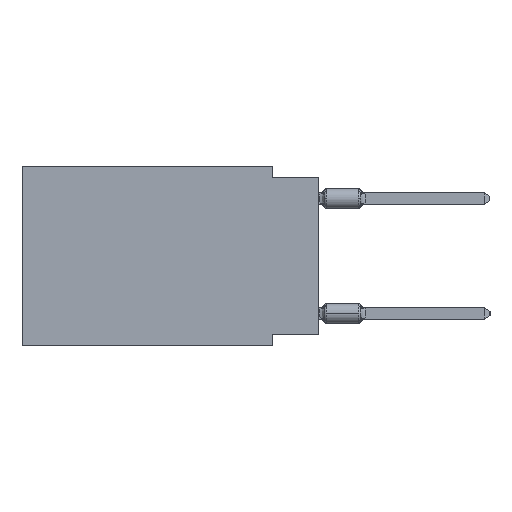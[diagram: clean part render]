
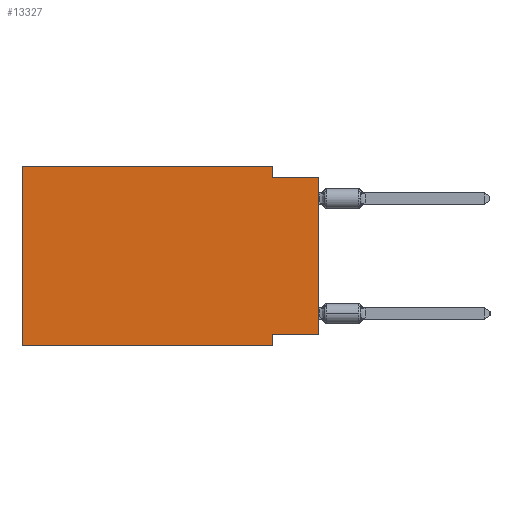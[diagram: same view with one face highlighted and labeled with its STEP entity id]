
A CAD part, left-side view. The second image highlights one B-rep face of the part: STEP entity #13327.
In plain terms, the highlighted planar face has unit normal (-1, 0, 0).
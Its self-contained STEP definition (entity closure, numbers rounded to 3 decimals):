
#387 = FACE_OUTER_BOUND ( 'NONE', #25145, .T. ) ;
#791 = ORIENTED_EDGE ( 'NONE', *, *, #5708, .F. ) ;
#1236 = VERTEX_POINT ( 'NONE', #37224 ) ;
#4182 = VERTEX_POINT ( 'NONE', #37004 ) ;
#5708 = EDGE_CURVE ( 'NONE', #1236, #16006, #26654, .T. ) ;
#6203 = CARTESIAN_POINT ( 'NONE',  ( 0., 2.54, -0.635 ) ) ;
#6431 = CARTESIAN_POINT ( 'NONE',  ( 0., 0., -0.635 ) ) ;
#6839 = CARTESIAN_POINT ( 'NONE',  ( 0., 16.383, 0. ) ) ;
#7902 = EDGE_CURVE ( 'NONE', #4182, #33020, #29954, .T. ) ;
#8092 = EDGE_CURVE ( 'NONE', #33118, #31930, #32764, .T. ) ;
#8436 = CARTESIAN_POINT ( 'NONE',  ( 0., 2.54, 0. ) ) ;
#8637 = CARTESIAN_POINT ( 'NONE',  ( 0., 0., 0. ) ) ;
#9473 = EDGE_CURVE ( 'NONE', #4182, #40887, #28924, .T. ) ;
#11282 = CARTESIAN_POINT ( 'NONE',  ( 0., 16.383, -9.906 ) ) ;
#11376 = DIRECTION ( 'NONE',  ( 0., -1., 0. ) ) ;
#12548 = VECTOR ( 'NONE', #14332, 1000. ) ;
#13201 = VECTOR ( 'NONE', #37579, 1000. ) ;
#13327 = ADVANCED_FACE ( 'NONE', ( #387 ), #26116, .F. ) ;
#13481 = EDGE_CURVE ( 'NONE', #31930, #33020, #23906, .T. ) ;
#14332 = DIRECTION ( 'NONE',  ( 0., 1., 0. ) ) ;
#16006 = VERTEX_POINT ( 'NONE', #6203 ) ;
#17047 = VECTOR ( 'NONE', #23444, 1000. ) ;
#17762 = DIRECTION ( 'NONE',  ( 0., 0., -1. ) ) ;
#18129 = EDGE_CURVE ( 'NONE', #33118, #28174, #41409, .T. ) ;
#19468 = VECTOR ( 'NONE', #34699, 1000. ) ;
#20542 = AXIS2_PLACEMENT_3D ( 'NONE', #29278, #29990, #44806 ) ;
#21072 = CARTESIAN_POINT ( 'NONE',  ( 0., 2.54, -9.906 ) ) ;
#21164 = DIRECTION ( 'NONE',  ( 0., 0., 1. ) ) ;
#21398 = CARTESIAN_POINT ( 'NONE',  ( 0., 2.54, -9.906 ) ) ;
#22075 = CARTESIAN_POINT ( 'NONE',  ( 0., 0., -9.271 ) ) ;
#22562 = DIRECTION ( 'NONE',  ( 0., -1., 0. ) ) ;
#23444 = DIRECTION ( 'NONE',  ( 0., 0., 1. ) ) ;
#23906 = LINE ( 'NONE', #21398, #38339 ) ;
#24475 = CARTESIAN_POINT ( 'NONE',  ( 0., 2.54, -9.271 ) ) ;
#25145 = EDGE_LOOP ( 'NONE', ( #28359, #39934, #791, #42863, #33775, #38544, #31518, #33280 ) ) ;
#26116 = PLANE ( 'NONE',  #20542 ) ;
#26191 = LINE ( 'NONE', #40520, #45864 ) ;
#26654 = LINE ( 'NONE', #8436, #13201 ) ;
#27417 = EDGE_CURVE ( 'NONE', #40887, #1236, #30040, .T. ) ;
#28174 = VERTEX_POINT ( 'NONE', #6431 ) ;
#28359 = ORIENTED_EDGE ( 'NONE', *, *, #18129, .T. ) ;
#28924 = LINE ( 'NONE', #6839, #40533 ) ;
#29278 = CARTESIAN_POINT ( 'NONE',  ( 0., 16.383, 0. ) ) ;
#29954 = LINE ( 'NONE', #11282, #19468 ) ;
#29990 = DIRECTION ( 'NONE',  ( 1., 0., 0. ) ) ;
#30040 = LINE ( 'NONE', #30284, #37020 ) ;
#30284 = CARTESIAN_POINT ( 'NONE',  ( 0., 16.383, 0. ) ) ;
#31518 = ORIENTED_EDGE ( 'NONE', *, *, #13481, .F. ) ;
#31930 = VERTEX_POINT ( 'NONE', #24475 ) ;
#32764 = LINE ( 'NONE', #22075, #12548 ) ;
#33020 = VERTEX_POINT ( 'NONE', #21072 ) ;
#33118 = VERTEX_POINT ( 'NONE', #47038 ) ;
#33280 = ORIENTED_EDGE ( 'NONE', *, *, #8092, .F. ) ;
#33775 = ORIENTED_EDGE ( 'NONE', *, *, #9473, .F. ) ;
#34699 = DIRECTION ( 'NONE',  ( 0., -1., 0. ) ) ;
#37004 = CARTESIAN_POINT ( 'NONE',  ( 0., 16.383, -9.906 ) ) ;
#37020 = VECTOR ( 'NONE', #11376, 1000. ) ;
#37224 = CARTESIAN_POINT ( 'NONE',  ( 0., 2.54, 0. ) ) ;
#37579 = DIRECTION ( 'NONE',  ( 0., 0., -1. ) ) ;
#38339 = VECTOR ( 'NONE', #17762, 1000. ) ;
#38544 = ORIENTED_EDGE ( 'NONE', *, *, #7902, .T. ) ;
#38790 = CARTESIAN_POINT ( 'NONE',  ( 0., 16.383, 0. ) ) ;
#39412 = EDGE_CURVE ( 'NONE', #16006, #28174, #26191, .T. ) ;
#39934 = ORIENTED_EDGE ( 'NONE', *, *, #39412, .F. ) ;
#40520 = CARTESIAN_POINT ( 'NONE',  ( 0., 0., -0.635 ) ) ;
#40533 = VECTOR ( 'NONE', #21164, 1000. ) ;
#40887 = VERTEX_POINT ( 'NONE', #38790 ) ;
#41409 = LINE ( 'NONE', #8637, #17047 ) ;
#42863 = ORIENTED_EDGE ( 'NONE', *, *, #27417, .F. ) ;
#44806 = DIRECTION ( 'NONE',  ( 0., 0., -1. ) ) ;
#45864 = VECTOR ( 'NONE', #22562, 1000. ) ;
#47038 = CARTESIAN_POINT ( 'NONE',  ( 0., 0., -9.271 ) ) ;
